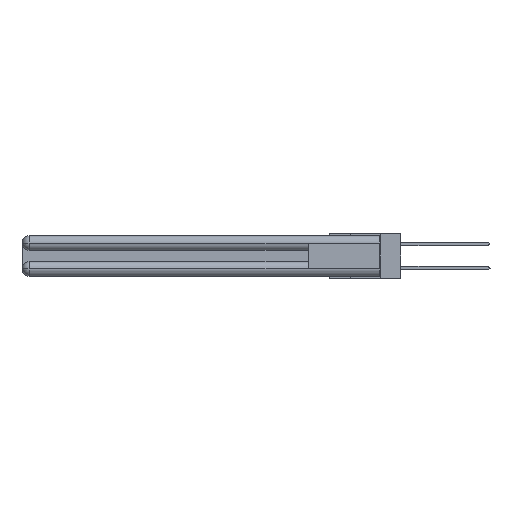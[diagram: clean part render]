
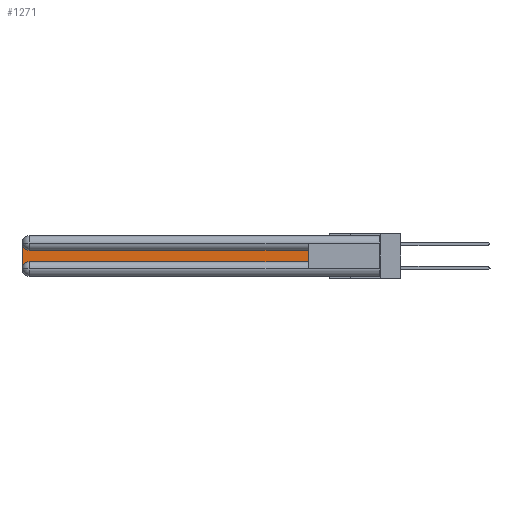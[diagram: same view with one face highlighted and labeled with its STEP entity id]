
A CAD part, left-side view. The second image highlights one B-rep face of the part: STEP entity #1271.
In plain terms, the highlighted planar face has unit normal (-1, 0, 0).
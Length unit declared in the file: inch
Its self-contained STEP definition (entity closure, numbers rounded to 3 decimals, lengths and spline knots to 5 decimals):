
#28 = EDGE_CURVE ( 'NONE', #15730, #27706, #10929, .T. ) ;
#129 = VERTEX_POINT ( 'NONE', #7827 ) ;
#1049 = CARTESIAN_POINT ( 'NONE',  ( 0.075, 0.6, -0.2175 ) ) ;
#1271 = ADVANCED_FACE ( 'NONE', ( #12348 ), #19621, .F. ) ;
#1900 = ORIENTED_EDGE ( 'NONE', *, *, #19946, .T. ) ;
#2038 = CIRCLE ( 'NONE', #25707, 0.06 ) ;
#2394 = VECTOR ( 'NONE', #16881, 39.37008 ) ;
#3085 = EDGE_CURVE ( 'NONE', #129, #15730, #21132, .T. ) ;
#3448 = ORIENTED_EDGE ( 'NONE', *, *, #28, .T. ) ;
#5480 = AXIS2_PLACEMENT_3D ( 'NONE', #10110, #12481, #22323 ) ;
#6199 = CARTESIAN_POINT ( 'NONE',  ( 0.075, 2.94, -0.0625 ) ) ;
#6979 = CARTESIAN_POINT ( 'NONE',  ( 0.075, 2.94, -0.2775 ) ) ;
#7179 = ORIENTED_EDGE ( 'NONE', *, *, #14636, .T. ) ;
#7827 = CARTESIAN_POINT ( 'NONE',  ( 0.075, 2.94, -0.2175 ) ) ;
#9762 = VECTOR ( 'NONE', #10957, 39.37008 ) ;
#10110 = CARTESIAN_POINT ( 'NONE',  ( 0.075, 3., -0.1225 ) ) ;
#10212 = CIRCLE ( 'NONE', #19398, 0.06 ) ;
#10929 = LINE ( 'NONE', #14642, #13183 ) ;
#10957 = DIRECTION ( 'NONE',  ( 0., 1., 0. ) ) ;
#11324 = LINE ( 'NONE', #26608, #2394 ) ;
#11940 = VERTEX_POINT ( 'NONE', #24402 ) ;
#12039 = VERTEX_POINT ( 'NONE', #26038 ) ;
#12348 = FACE_OUTER_BOUND ( 'NONE', #26131, .T. ) ;
#12481 = DIRECTION ( 'NONE',  ( 1., 0., 0. ) ) ;
#13095 = ORIENTED_EDGE ( 'NONE', *, *, #3085, .T. ) ;
#13183 = VECTOR ( 'NONE', #21707, 39.37008 ) ;
#14636 = EDGE_CURVE ( 'NONE', #27706, #21704, #17544, .T. ) ;
#14642 = CARTESIAN_POINT ( 'NONE',  ( 0.075, 0.6, -0.2175 ) ) ;
#15730 = VERTEX_POINT ( 'NONE', #1049 ) ;
#16298 = CARTESIAN_POINT ( 'NONE',  ( 0.075, 2.94, -0.1225 ) ) ;
#16881 = DIRECTION ( 'NONE',  ( 0., 0., -1. ) ) ;
#17544 = LINE ( 'NONE', #20581, #9762 ) ;
#18290 = EDGE_CURVE ( 'NONE', #11940, #12039, #11324, .T. ) ;
#18608 = DIRECTION ( 'NONE',  ( 0., 0., -1. ) ) ;
#19398 = AXIS2_PLACEMENT_3D ( 'NONE', #6199, #27360, #27451 ) ;
#19621 = PLANE ( 'NONE',  #5480 ) ;
#19946 = EDGE_CURVE ( 'NONE', #21704, #11940, #10212, .T. ) ;
#20098 = DIRECTION ( 'NONE',  ( 0., -1., 0. ) ) ;
#20581 = CARTESIAN_POINT ( 'NONE',  ( 0.075, 0.6, -0.1225 ) ) ;
#21132 = LINE ( 'NONE', #26926, #25184 ) ;
#21704 = VERTEX_POINT ( 'NONE', #16298 ) ;
#21707 = DIRECTION ( 'NONE',  ( 0., 0., 1. ) ) ;
#22323 = DIRECTION ( 'NONE',  ( 0., 0., -1. ) ) ;
#24402 = CARTESIAN_POINT ( 'NONE',  ( 0.075, 3., -0.0625 ) ) ;
#25184 = VECTOR ( 'NONE', #20098, 39.37008 ) ;
#25707 = AXIS2_PLACEMENT_3D ( 'NONE', #6979, #25935, #18608 ) ;
#25755 = CARTESIAN_POINT ( 'NONE',  ( 0.075, 0.6, -0.1225 ) ) ;
#25935 = DIRECTION ( 'NONE',  ( 1., 0., 0. ) ) ;
#26038 = CARTESIAN_POINT ( 'NONE',  ( 0.075, 3., -0.2775 ) ) ;
#26131 = EDGE_LOOP ( 'NONE', ( #7179, #1900, #29155, #28368, #13095, #3448 ) ) ;
#26608 = CARTESIAN_POINT ( 'NONE',  ( 0.075, 3., -0.2175 ) ) ;
#26926 = CARTESIAN_POINT ( 'NONE',  ( 0.075, 0.6, -0.2175 ) ) ;
#27360 = DIRECTION ( 'NONE',  ( 1., 0., 0. ) ) ;
#27451 = DIRECTION ( 'NONE',  ( 0., 0., -1. ) ) ;
#27706 = VERTEX_POINT ( 'NONE', #25755 ) ;
#28368 = ORIENTED_EDGE ( 'NONE', *, *, #28711, .T. ) ;
#28711 = EDGE_CURVE ( 'NONE', #12039, #129, #2038, .T. ) ;
#29155 = ORIENTED_EDGE ( 'NONE', *, *, #18290, .T. ) ;
